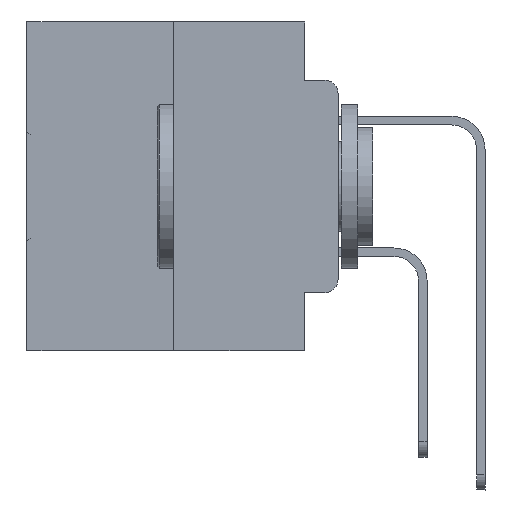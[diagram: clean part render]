
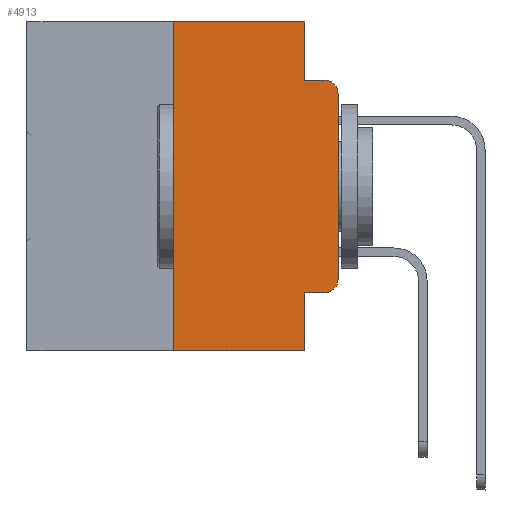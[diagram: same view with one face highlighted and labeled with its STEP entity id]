
A CAD part, left-side view. The second image highlights one B-rep face of the part: STEP entity #4913.
In plain terms, the highlighted planar face has unit normal (-1, 0, 0).
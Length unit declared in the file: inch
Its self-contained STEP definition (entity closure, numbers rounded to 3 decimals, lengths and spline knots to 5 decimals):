
#62 = CARTESIAN_POINT ( 'NONE',  ( 0., 0.051, -0.5 ) ) ;
#80 = DIRECTION ( 'NONE',  ( 0., 0., -1. ) ) ;
#487 = CARTESIAN_POINT ( 'NONE',  ( 0., 0.473, 0. ) ) ;
#1698 = AXIS2_PLACEMENT_3D ( 'NONE', #27753, #3281, #25087 ) ;
#1717 = VERTEX_POINT ( 'NONE', #31793 ) ;
#2363 = EDGE_CURVE ( 'NONE', #13557, #13867, #8479, .T. ) ;
#2611 = VECTOR ( 'NONE', #9910, 39.37008 ) ;
#3281 = DIRECTION ( 'NONE',  ( -1., 0., 0. ) ) ;
#3335 = VECTOR ( 'NONE', #19396, 39.37008 ) ;
#3798 = VERTEX_POINT ( 'NONE', #13594 ) ;
#3910 = VERTEX_POINT ( 'NONE', #28438 ) ;
#4220 = LINE ( 'NONE', #23519, #6266 ) ;
#4477 = CARTESIAN_POINT ( 'NONE',  ( 0., 0.051, 0. ) ) ;
#4712 = DIRECTION ( 'NONE',  ( 0., -1., 0. ) ) ;
#4719 = ORIENTED_EDGE ( 'NONE', *, *, #30149, .T. ) ;
#4913 = ADVANCED_FACE ( 'NONE', ( #6202 ), #33363, .F. ) ;
#6202 = FACE_OUTER_BOUND ( 'NONE', #8411, .T. ) ;
#6260 = CIRCLE ( 'NONE', #1698, 0.02 ) ;
#6266 = VECTOR ( 'NONE', #9751, 39.37008 ) ;
#6617 = ORIENTED_EDGE ( 'NONE', *, *, #26478, .F. ) ;
#8275 = ORIENTED_EDGE ( 'NONE', *, *, #2363, .F. ) ;
#8290 = EDGE_CURVE ( 'NONE', #10544, #3910, #9046, .T. ) ;
#8369 = AXIS2_PLACEMENT_3D ( 'NONE', #487, #11364, #25145 ) ;
#8411 = EDGE_LOOP ( 'NONE', ( #20944, #10120, #13770, #28751, #6617, #22330, #18481, #8275, #27102, #4719 ) ) ;
#8479 = LINE ( 'NONE', #17736, #3335 ) ;
#8513 = VECTOR ( 'NONE', #4712, 39.37008 ) ;
#8814 = EDGE_CURVE ( 'NONE', #1717, #33095, #6260, .T. ) ;
#8967 = CARTESIAN_POINT ( 'NONE',  ( 0., 0.25, -0.5 ) ) ;
#9046 = LINE ( 'NONE', #14203, #18576 ) ;
#9749 = VECTOR ( 'NONE', #21083, 39.37008 ) ;
#9751 = DIRECTION ( 'NONE',  ( 0., -1., 0. ) ) ;
#9910 = DIRECTION ( 'NONE',  ( 0., -1., 0. ) ) ;
#9971 = LINE ( 'NONE', #29243, #18043 ) ;
#10120 = ORIENTED_EDGE ( 'NONE', *, *, #8814, .T. ) ;
#10544 = VERTEX_POINT ( 'NONE', #8967 ) ;
#11364 = DIRECTION ( 'NONE',  ( 1., 0., 0. ) ) ;
#11509 = CARTESIAN_POINT ( 'NONE',  ( 0., 0.051, -0.4115 ) ) ;
#11525 = DIRECTION ( 'NONE',  ( 0., 0., 1. ) ) ;
#11941 = AXIS2_PLACEMENT_3D ( 'NONE', #16685, #27218, #80 ) ;
#13557 = VERTEX_POINT ( 'NONE', #11509 ) ;
#13594 = CARTESIAN_POINT ( 'NONE',  ( 0., 0.051, -0.0885 ) ) ;
#13770 = ORIENTED_EDGE ( 'NONE', *, *, #19978, .F. ) ;
#13867 = VERTEX_POINT ( 'NONE', #62 ) ;
#14020 = VERTEX_POINT ( 'NONE', #28278 ) ;
#14203 = CARTESIAN_POINT ( 'NONE',  ( 0., 0.25, 0. ) ) ;
#14643 = DIRECTION ( 'NONE',  ( 0., 0., -1. ) ) ;
#15197 = CARTESIAN_POINT ( 'NONE',  ( 0., 0.051, -0.0885 ) ) ;
#16685 = CARTESIAN_POINT ( 'NONE',  ( 0., 0.02, -0.3915 ) ) ;
#16739 = VERTEX_POINT ( 'NONE', #25036 ) ;
#17736 = CARTESIAN_POINT ( 'NONE',  ( 0., 0.051, 0. ) ) ;
#18043 = VECTOR ( 'NONE', #23224, 39.37008 ) ;
#18116 = CARTESIAN_POINT ( 'NONE',  ( 0., 0.051, -0.4115 ) ) ;
#18481 = ORIENTED_EDGE ( 'NONE', *, *, #31194, .T. ) ;
#18576 = VECTOR ( 'NONE', #11525, 39.37008 ) ;
#18676 = EDGE_CURVE ( 'NONE', #16739, #1717, #9971, .T. ) ;
#19396 = DIRECTION ( 'NONE',  ( 0., 0., -1. ) ) ;
#19509 = VERTEX_POINT ( 'NONE', #4477 ) ;
#19978 = EDGE_CURVE ( 'NONE', #3798, #33095, #28768, .T. ) ;
#20944 = ORIENTED_EDGE ( 'NONE', *, *, #18676, .T. ) ;
#21083 = DIRECTION ( 'NONE',  ( 0., -1., 0. ) ) ;
#22330 = ORIENTED_EDGE ( 'NONE', *, *, #8290, .F. ) ;
#22701 = CARTESIAN_POINT ( 'NONE',  ( 0., 0.051, 0. ) ) ;
#23224 = DIRECTION ( 'NONE',  ( 0., 0., 1. ) ) ;
#23519 = CARTESIAN_POINT ( 'NONE',  ( 0., 0.473, -0.5 ) ) ;
#25036 = CARTESIAN_POINT ( 'NONE',  ( 0., 0., -0.3915 ) ) ;
#25087 = DIRECTION ( 'NONE',  ( 0., 0., -1. ) ) ;
#25145 = DIRECTION ( 'NONE',  ( 0., 0., -1. ) ) ;
#26210 = CIRCLE ( 'NONE', #11941, 0.02 ) ;
#26478 = EDGE_CURVE ( 'NONE', #3910, #19509, #34393, .T. ) ;
#27102 = ORIENTED_EDGE ( 'NONE', *, *, #32595, .T. ) ;
#27218 = DIRECTION ( 'NONE',  ( -1., 0., 0. ) ) ;
#27753 = CARTESIAN_POINT ( 'NONE',  ( 0., 0.02, -0.1085 ) ) ;
#28278 = CARTESIAN_POINT ( 'NONE',  ( 0., 0.02, -0.4115 ) ) ;
#28438 = CARTESIAN_POINT ( 'NONE',  ( 0., 0.25, 0. ) ) ;
#28751 = ORIENTED_EDGE ( 'NONE', *, *, #33255, .F. ) ;
#28768 = LINE ( 'NONE', #15197, #9749 ) ;
#29243 = CARTESIAN_POINT ( 'NONE',  ( 0., 0., 0. ) ) ;
#29651 = VECTOR ( 'NONE', #14643, 39.37008 ) ;
#30149 = EDGE_CURVE ( 'NONE', #14020, #16739, #26210, .T. ) ;
#31194 = EDGE_CURVE ( 'NONE', #10544, #13867, #4220, .T. ) ;
#31704 = LINE ( 'NONE', #18116, #8513 ) ;
#31793 = CARTESIAN_POINT ( 'NONE',  ( 0., 0., -0.1085 ) ) ;
#32595 = EDGE_CURVE ( 'NONE', #13557, #14020, #31704, .T. ) ;
#32690 = CARTESIAN_POINT ( 'NONE',  ( 0., 0.02, -0.0885 ) ) ;
#33095 = VERTEX_POINT ( 'NONE', #32690 ) ;
#33255 = EDGE_CURVE ( 'NONE', #19509, #3798, #33410, .T. ) ;
#33363 = PLANE ( 'NONE',  #8369 ) ;
#33410 = LINE ( 'NONE', #22701, #29651 ) ;
#34393 = LINE ( 'NONE', #34734, #2611 ) ;
#34734 = CARTESIAN_POINT ( 'NONE',  ( 0., 0.473, 0. ) ) ;
